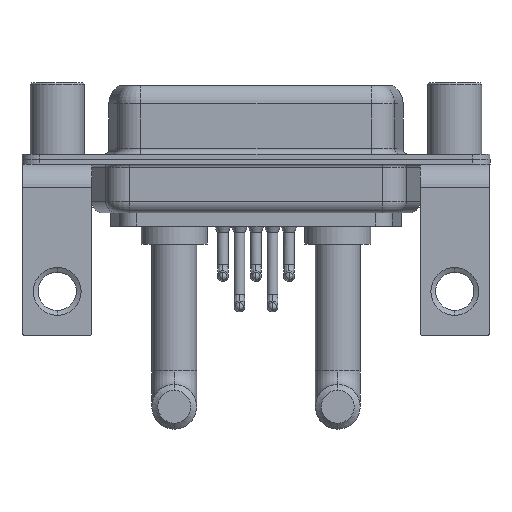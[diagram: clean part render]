
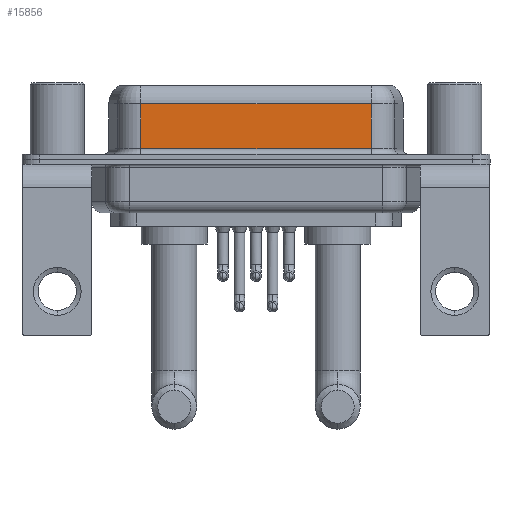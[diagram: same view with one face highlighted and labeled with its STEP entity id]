
A CAD part, front view. The second image highlights one B-rep face of the part: STEP entity #15856.
In plain terms, the highlighted planar face has unit normal (0, -1, 0).
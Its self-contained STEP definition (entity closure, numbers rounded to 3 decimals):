
#923 = ORIENTED_EDGE ( 'NONE', *, *, #16027, .T. ) ;
#1427 = LINE ( 'NONE', #7424, #3742 ) ;
#2203 = VERTEX_POINT ( 'NONE', #3961 ) ;
#2761 = CARTESIAN_POINT ( 'NONE',  ( 7.013, -3.95, 6.4 ) ) ;
#3100 = EDGE_CURVE ( 'NONE', #5823, #2203, #10098, .T. ) ;
#3157 = CARTESIAN_POINT ( 'NONE',  ( 7.013, -3.95, 0.9 ) ) ;
#3363 = CARTESIAN_POINT ( 'NONE',  ( 26.287, -3.95, 4.65 ) ) ;
#3742 = VECTOR ( 'NONE', #13397, 1000. ) ;
#3913 = EDGE_CURVE ( 'NONE', #14302, #5667, #11498, .T. ) ;
#3961 = CARTESIAN_POINT ( 'NONE',  ( 26.287, -3.95, 0.9 ) ) ;
#4169 = CARTESIAN_POINT ( 'NONE',  ( 7.013, -3.95, 4.65 ) ) ;
#4191 = PLANE ( 'NONE',  #19092 ) ;
#5442 = VECTOR ( 'NONE', #14735, 1000. ) ;
#5502 = CARTESIAN_POINT ( 'NONE',  ( 26.287, -3.95, 6.4 ) ) ;
#5667 = VERTEX_POINT ( 'NONE', #3157 ) ;
#5823 = VERTEX_POINT ( 'NONE', #3363 ) ;
#5976 = CARTESIAN_POINT ( 'NONE',  ( 26.287, -3.95, 6.4 ) ) ;
#7346 = DIRECTION ( 'NONE',  ( 0., 1., 0. ) ) ;
#7424 = CARTESIAN_POINT ( 'NONE',  ( 26.287, -3.95, 0.9 ) ) ;
#7954 = EDGE_LOOP ( 'NONE', ( #10173, #923, #18736, #13805 ) ) ;
#10098 = LINE ( 'NONE', #5502, #17575 ) ;
#10173 = ORIENTED_EDGE ( 'NONE', *, *, #3100, .F. ) ;
#10961 = DIRECTION ( 'NONE',  ( -1., 0., 0. ) ) ;
#11498 = LINE ( 'NONE', #2761, #5442 ) ;
#12140 = LINE ( 'NONE', #18212, #16267 ) ;
#12652 = DIRECTION ( 'NONE',  ( 0., 0., -1. ) ) ;
#13324 = DIRECTION ( 'NONE',  ( 0., 0., 1. ) ) ;
#13397 = DIRECTION ( 'NONE',  ( 1., 0., 0. ) ) ;
#13805 = ORIENTED_EDGE ( 'NONE', *, *, #16490, .T. ) ;
#14302 = VERTEX_POINT ( 'NONE', #4169 ) ;
#14735 = DIRECTION ( 'NONE',  ( 0., 0., -1. ) ) ;
#15856 = ADVANCED_FACE ( 'NONE', ( #16351 ), #4191, .F. ) ;
#16027 = EDGE_CURVE ( 'NONE', #5823, #14302, #12140, .T. ) ;
#16267 = VECTOR ( 'NONE', #10961, 1000. ) ;
#16351 = FACE_OUTER_BOUND ( 'NONE', #7954, .T. ) ;
#16490 = EDGE_CURVE ( 'NONE', #5667, #2203, #1427, .T. ) ;
#17575 = VECTOR ( 'NONE', #12652, 1000. ) ;
#18212 = CARTESIAN_POINT ( 'NONE',  ( 26.287, -3.95, 4.65 ) ) ;
#18736 = ORIENTED_EDGE ( 'NONE', *, *, #3913, .T. ) ;
#19092 = AXIS2_PLACEMENT_3D ( 'NONE', #5976, #7346, #13324 ) ;
